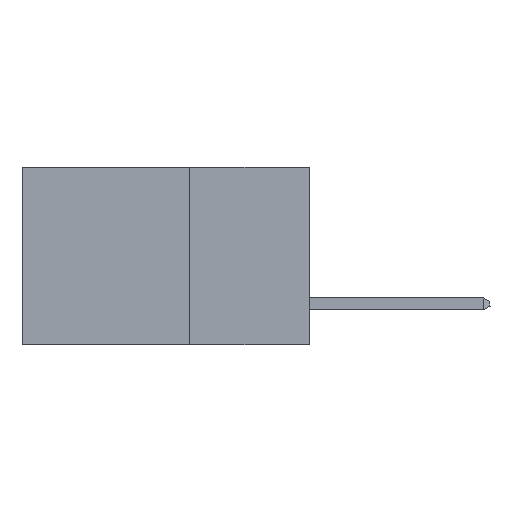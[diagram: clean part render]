
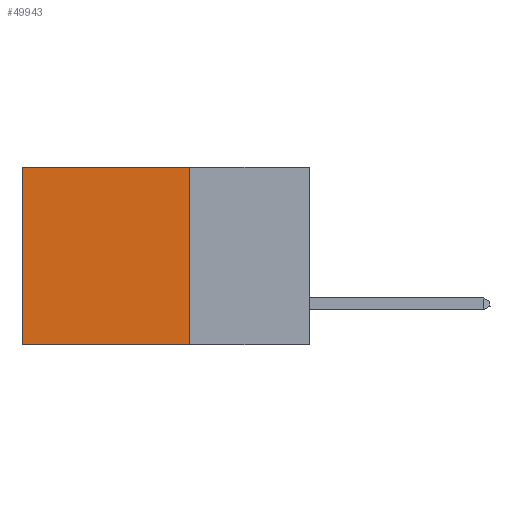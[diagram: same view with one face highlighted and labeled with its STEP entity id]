
A CAD part, left-side view. The second image highlights one B-rep face of the part: STEP entity #49943.
In plain terms, the highlighted planar face has unit normal (-1, 0, 0).
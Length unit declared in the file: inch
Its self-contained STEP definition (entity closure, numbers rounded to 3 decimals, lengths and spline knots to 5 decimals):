
#732 = CARTESIAN_POINT ( 'NONE',  ( 0.2875, 0.6, 0. ) ) ;
#797 = VERTEX_POINT ( 'NONE', #6194 ) ;
#1577 = DIRECTION ( 'NONE',  ( 0., 1., 0. ) ) ;
#3603 = EDGE_CURVE ( 'NONE', #14309, #32317, #18111, .T. ) ;
#4000 = CARTESIAN_POINT ( 'NONE',  ( 0.2875, 0.25, -0.37 ) ) ;
#4482 = DIRECTION ( 'NONE',  ( 0., 0., -1. ) ) ;
#5615 = VERTEX_POINT ( 'NONE', #37933 ) ;
#5756 = EDGE_CURVE ( 'NONE', #14309, #797, #46915, .T. ) ;
#6194 = CARTESIAN_POINT ( 'NONE',  ( 0.2875, 0.25, -0.37 ) ) ;
#6286 = ORIENTED_EDGE ( 'NONE', *, *, #37236, .F. ) ;
#8859 = EDGE_CURVE ( 'NONE', #32317, #5615, #48264, .T. ) ;
#11615 = CARTESIAN_POINT ( 'NONE',  ( 0.2875, 0.25, 0. ) ) ;
#12412 = ORIENTED_EDGE ( 'NONE', *, *, #3603, .T. ) ;
#14309 = VERTEX_POINT ( 'NONE', #20315 ) ;
#15479 = PLANE ( 'NONE',  #27171 ) ;
#18111 = LINE ( 'NONE', #47898, #46475 ) ;
#19331 = CARTESIAN_POINT ( 'NONE',  ( 0.2875, 0.25, 0. ) ) ;
#20315 = CARTESIAN_POINT ( 'NONE',  ( 0.2875, 0.25, 0. ) ) ;
#20640 = ORIENTED_EDGE ( 'NONE', *, *, #5756, .F. ) ;
#23174 = DIRECTION ( 'NONE',  ( 0., 0., -1. ) ) ;
#23243 = DIRECTION ( 'NONE',  ( 0., 0., -1. ) ) ;
#26742 = LINE ( 'NONE', #4000, #35807 ) ;
#27171 = AXIS2_PLACEMENT_3D ( 'NONE', #19331, #46297, #23174 ) ;
#27225 = DIRECTION ( 'NONE',  ( 0., 1., 0. ) ) ;
#32317 = VERTEX_POINT ( 'NONE', #732 ) ;
#33679 = EDGE_LOOP ( 'NONE', ( #45685, #6286, #20640, #12412 ) ) ;
#35807 = VECTOR ( 'NONE', #27225, 39.37008 ) ;
#37236 = EDGE_CURVE ( 'NONE', #797, #5615, #26742, .T. ) ;
#37933 = CARTESIAN_POINT ( 'NONE',  ( 0.2875, 0.6, -0.37 ) ) ;
#38026 = VECTOR ( 'NONE', #4482, 39.37008 ) ;
#39168 = CARTESIAN_POINT ( 'NONE',  ( 0.2875, 0.6, 0. ) ) ;
#42521 = FACE_OUTER_BOUND ( 'NONE', #33679, .T. ) ;
#45685 = ORIENTED_EDGE ( 'NONE', *, *, #8859, .T. ) ;
#45705 = VECTOR ( 'NONE', #23243, 39.37008 ) ;
#46297 = DIRECTION ( 'NONE',  ( 1., 0., 0. ) ) ;
#46475 = VECTOR ( 'NONE', #1577, 39.37008 ) ;
#46915 = LINE ( 'NONE', #11615, #45705 ) ;
#47898 = CARTESIAN_POINT ( 'NONE',  ( 0.2875, 0.25, 0. ) ) ;
#48264 = LINE ( 'NONE', #39168, #38026 ) ;
#49943 = ADVANCED_FACE ( 'NONE', ( #42521 ), #15479, .F. ) ;
